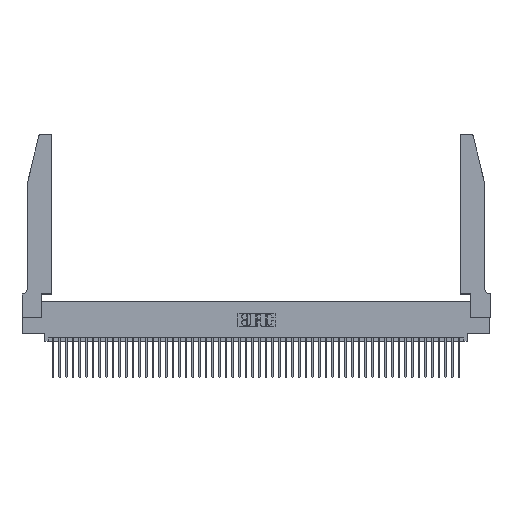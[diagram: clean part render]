
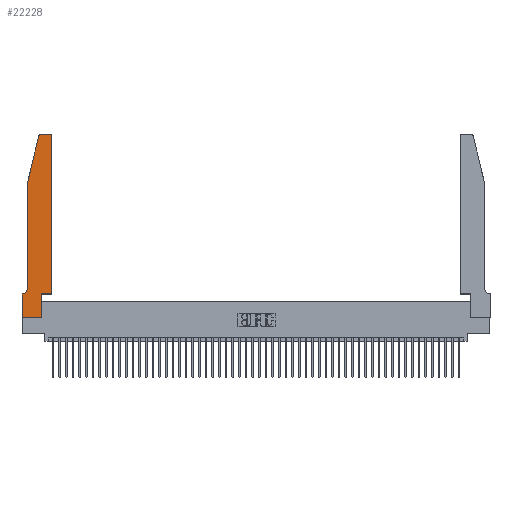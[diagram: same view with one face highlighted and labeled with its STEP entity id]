
A CAD part, top view. The second image highlights one B-rep face of the part: STEP entity #22228.
In plain terms, the highlighted planar face has unit normal (0, 0, 1).
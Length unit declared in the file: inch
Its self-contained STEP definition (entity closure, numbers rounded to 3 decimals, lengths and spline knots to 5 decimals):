
#64 = CARTESIAN_POINT ( 'NONE',  ( 0., 0., 0.37 ) ) ;
#208 = VERTEX_POINT ( 'NONE', #31436 ) ;
#616 = VECTOR ( 'NONE', #36595, 39.37008 ) ;
#1802 = EDGE_CURVE ( 'NONE', #208, #48669, #41471, .T. ) ;
#2058 = EDGE_CURVE ( 'NONE', #43197, #30878, #22515, .T. ) ;
#3596 = VERTEX_POINT ( 'NONE', #29754 ) ;
#4964 = DIRECTION ( 'NONE',  ( 1., 0., 0. ) ) ;
#5848 = CARTESIAN_POINT ( 'NONE',  ( 0.4505, 0.35, 0.37 ) ) ;
#6301 = CARTESIAN_POINT ( 'NONE',  ( 0., 0.35, 0.37 ) ) ;
#6410 = CARTESIAN_POINT ( 'NONE',  ( 0.0055, 0.35, 0.37 ) ) ;
#6890 = LINE ( 'NONE', #40778, #27905 ) ;
#7826 = CARTESIAN_POINT ( 'NONE',  ( 0.0755, 2., 0.37 ) ) ;
#8128 = PLANE ( 'NONE',  #27025 ) ;
#8497 = EDGE_CURVE ( 'NONE', #14591, #25457, #45774, .T. ) ;
#9009 = CARTESIAN_POINT ( 'NONE',  ( 0., 0., 0.37 ) ) ;
#9257 = ORIENTED_EDGE ( 'NONE', *, *, #14369, .T. ) ;
#10127 = DIRECTION ( 'NONE',  ( 0., 0., 1. ) ) ;
#10447 = VECTOR ( 'NONE', #4964, 39.37008 ) ;
#10692 = EDGE_LOOP ( 'NONE', ( #22601, #45795, #38594, #49885, #14883, #19544, #42950, #30072, #9257, #12735, #47370, #20305 ) ) ;
#10926 = AXIS2_PLACEMENT_3D ( 'NONE', #20148, #47395, #24097 ) ;
#11310 = LINE ( 'NONE', #40371, #616 ) ;
#11347 = VECTOR ( 'NONE', #43188, 39.37008 ) ;
#11853 = CARTESIAN_POINT ( 'NONE',  ( 0.25487, 2.72718, 0.37 ) ) ;
#12310 = DIRECTION ( 'NONE',  ( 1., 0., 0. ) ) ;
#12735 = ORIENTED_EDGE ( 'NONE', *, *, #37531, .T. ) ;
#12940 = EDGE_CURVE ( 'NONE', #48669, #42240, #30760, .T. ) ;
#13168 = CARTESIAN_POINT ( 'NONE',  ( 0.2605, 2.75, 0.37 ) ) ;
#13373 = VECTOR ( 'NONE', #27808, 39.37008 ) ;
#13709 = CARTESIAN_POINT ( 'NONE',  ( 0.4205, 2.75, 0.37 ) ) ;
#14369 = EDGE_CURVE ( 'NONE', #3596, #33878, #11310, .T. ) ;
#14591 = VERTEX_POINT ( 'NONE', #6301 ) ;
#14816 = CARTESIAN_POINT ( 'NONE',  ( 0.4205, 2.72, 0.37 ) ) ;
#14883 = ORIENTED_EDGE ( 'NONE', *, *, #2058, .T. ) ;
#15256 = CARTESIAN_POINT ( 'NONE',  ( 0.0755, 0.35, 0.37 ) ) ;
#15734 = EDGE_CURVE ( 'NONE', #27435, #47894, #49139, .T. ) ;
#15952 = CIRCLE ( 'NONE', #35202, 0.03 ) ;
#17092 = EDGE_CURVE ( 'NONE', #25457, #3596, #20960, .T. ) ;
#18791 = DIRECTION ( 'NONE',  ( 1., 0., 0. ) ) ;
#19544 = ORIENTED_EDGE ( 'NONE', *, *, #39637, .T. ) ;
#19836 = AXIS2_PLACEMENT_3D ( 'NONE', #14816, #42212, #18791 ) ;
#20148 = CARTESIAN_POINT ( 'NONE',  ( 0.0055, 0.42, 0.37 ) ) ;
#20164 = CARTESIAN_POINT ( 'NONE',  ( 0.0755, 2., 0.37 ) ) ;
#20305 = ORIENTED_EDGE ( 'NONE', *, *, #1802, .T. ) ;
#20446 = CARTESIAN_POINT ( 'NONE',  ( 0.0755, 0.42, 0.37 ) ) ;
#20960 = LINE ( 'NONE', #40421, #10447 ) ;
#21814 = LINE ( 'NONE', #7826, #11347 ) ;
#22228 = ADVANCED_FACE ( 'NONE', ( #28515 ), #8128, .T. ) ;
#22515 = CIRCLE ( 'NONE', #10926, 0.07 ) ;
#22601 = ORIENTED_EDGE ( 'NONE', *, *, #12940, .T. ) ;
#22962 = LINE ( 'NONE', #15256, #30894 ) ;
#24097 = DIRECTION ( 'NONE',  ( -1., 0., 0. ) ) ;
#25457 = VERTEX_POINT ( 'NONE', #9009 ) ;
#27025 = AXIS2_PLACEMENT_3D ( 'NONE', #43465, #35767, #12310 ) ;
#27435 = VERTEX_POINT ( 'NONE', #11853 ) ;
#27808 = DIRECTION ( 'NONE',  ( 0., -1., 0. ) ) ;
#27905 = VECTOR ( 'NONE', #44650, 39.37008 ) ;
#28515 = FACE_OUTER_BOUND ( 'NONE', #10692, .T. ) ;
#29754 = CARTESIAN_POINT ( 'NONE',  ( 0.2865, 0., 0.37 ) ) ;
#30072 = ORIENTED_EDGE ( 'NONE', *, *, #17092, .T. ) ;
#30084 = CARTESIAN_POINT ( 'NONE',  ( 0.284, 2.75, 0.37 ) ) ;
#30760 = LINE ( 'NONE', #13168, #37459 ) ;
#30878 = VERTEX_POINT ( 'NONE', #6410 ) ;
#30894 = VECTOR ( 'NONE', #38698, 39.37008 ) ;
#31436 = CARTESIAN_POINT ( 'NONE',  ( 0.4505, 2.72, 0.37 ) ) ;
#33307 = VECTOR ( 'NONE', #37325, 39.37008 ) ;
#33635 = VERTEX_POINT ( 'NONE', #45860 ) ;
#33655 = CARTESIAN_POINT ( 'NONE',  ( 0.284, 2.72, 0.37 ) ) ;
#33878 = VERTEX_POINT ( 'NONE', #36148 ) ;
#35202 = AXIS2_PLACEMENT_3D ( 'NONE', #33655, #10127, #37565 ) ;
#35767 = DIRECTION ( 'NONE',  ( 0., 0., 1. ) ) ;
#36148 = CARTESIAN_POINT ( 'NONE',  ( 0.2865, 0.35, 0.37 ) ) ;
#36595 = DIRECTION ( 'NONE',  ( 0., 1., 0. ) ) ;
#36964 = EDGE_CURVE ( 'NONE', #33635, #208, #6890, .T. ) ;
#37325 = DIRECTION ( 'NONE',  ( 1., 0., 0. ) ) ;
#37459 = VECTOR ( 'NONE', #40577, 39.37008 ) ;
#37531 = EDGE_CURVE ( 'NONE', #33878, #33635, #43696, .T. ) ;
#37565 = DIRECTION ( 'NONE',  ( 1., 0., 0. ) ) ;
#38594 = ORIENTED_EDGE ( 'NONE', *, *, #15734, .T. ) ;
#38698 = DIRECTION ( 'NONE',  ( -1., 0., 0. ) ) ;
#39637 = EDGE_CURVE ( 'NONE', #30878, #14591, #22962, .T. ) ;
#40371 = CARTESIAN_POINT ( 'NONE',  ( 0.2865, 0.35, 0.37 ) ) ;
#40421 = CARTESIAN_POINT ( 'NONE',  ( 0., 0., 0.37 ) ) ;
#40577 = DIRECTION ( 'NONE',  ( -1., 0., 0. ) ) ;
#40778 = CARTESIAN_POINT ( 'NONE',  ( 0.4505, 0.35, 0.37 ) ) ;
#41471 = CIRCLE ( 'NONE', #19836, 0.03 ) ;
#41890 = VECTOR ( 'NONE', #48345, 39.37008 ) ;
#42212 = DIRECTION ( 'NONE',  ( 0., 0., 1. ) ) ;
#42240 = VERTEX_POINT ( 'NONE', #30084 ) ;
#42950 = ORIENTED_EDGE ( 'NONE', *, *, #8497, .T. ) ;
#43188 = DIRECTION ( 'NONE',  ( 0., -1., 0. ) ) ;
#43197 = VERTEX_POINT ( 'NONE', #20446 ) ;
#43465 = CARTESIAN_POINT ( 'NONE',  ( 0., 0.35, 0.37 ) ) ;
#43696 = LINE ( 'NONE', #5848, #33307 ) ;
#44475 = CARTESIAN_POINT ( 'NONE',  ( 0.0755, 2., 0.37 ) ) ;
#44650 = DIRECTION ( 'NONE',  ( 0., 1., 0. ) ) ;
#45774 = LINE ( 'NONE', #64, #13373 ) ;
#45795 = ORIENTED_EDGE ( 'NONE', *, *, #48020, .T. ) ;
#45860 = CARTESIAN_POINT ( 'NONE',  ( 0.4505, 0.35, 0.37 ) ) ;
#47370 = ORIENTED_EDGE ( 'NONE', *, *, #36964, .T. ) ;
#47395 = DIRECTION ( 'NONE',  ( 0., 0., -1. ) ) ;
#47894 = VERTEX_POINT ( 'NONE', #20164 ) ;
#48020 = EDGE_CURVE ( 'NONE', #42240, #27435, #15952, .T. ) ;
#48345 = DIRECTION ( 'NONE',  ( -0.239, -0.971, 0. ) ) ;
#48669 = VERTEX_POINT ( 'NONE', #13709 ) ;
#49139 = LINE ( 'NONE', #44475, #41890 ) ;
#49885 = ORIENTED_EDGE ( 'NONE', *, *, #50630, .T. ) ;
#50630 = EDGE_CURVE ( 'NONE', #47894, #43197, #21814, .T. ) ;
